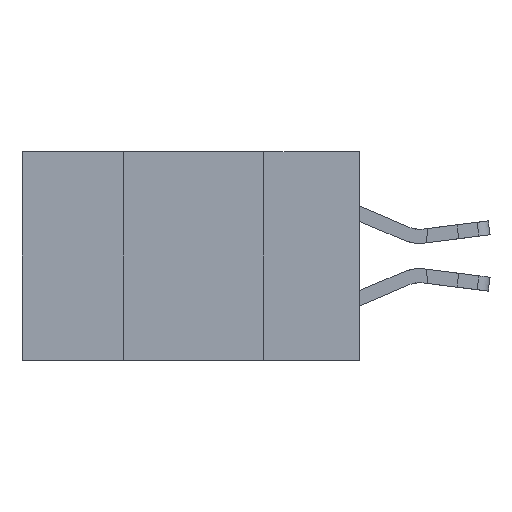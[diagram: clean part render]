
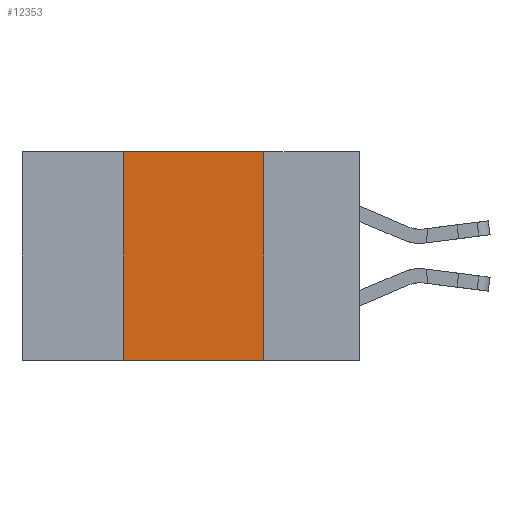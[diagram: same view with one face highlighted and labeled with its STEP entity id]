
A CAD part, left-side view. The second image highlights one B-rep face of the part: STEP entity #12353.
In plain terms, the highlighted planar face has unit normal (-1, 0, 0).
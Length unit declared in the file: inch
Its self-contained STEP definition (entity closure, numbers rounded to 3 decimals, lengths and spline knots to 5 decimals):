
#75 = ORIENTED_EDGE ( 'NONE', *, *, #1564, .F. ) ;
#1560 = AXIS2_PLACEMENT_3D ( 'NONE', #17747, #12149, #10774 ) ;
#1564 = EDGE_CURVE ( 'NONE', #12366, #2827, #11663, .T. ) ;
#2827 = VERTEX_POINT ( 'NONE', #4999 ) ;
#3298 = CARTESIAN_POINT ( 'NONE',  ( 0., 0.6, -0.37 ) ) ;
#3664 = CARTESIAN_POINT ( 'NONE',  ( 0., 0.42, 0. ) ) ;
#4999 = CARTESIAN_POINT ( 'NONE',  ( 0., 0.42, 0. ) ) ;
#5420 = CARTESIAN_POINT ( 'NONE',  ( 0., 0.17, 0. ) ) ;
#5741 = VECTOR ( 'NONE', #18306, 39.37008 ) ;
#5853 = EDGE_LOOP ( 'NONE', ( #17055, #16620, #75, #18424 ) ) ;
#5972 = EDGE_CURVE ( 'NONE', #16258, #6497, #9578, .T. ) ;
#6440 = PLANE ( 'NONE',  #1560 ) ;
#6497 = VERTEX_POINT ( 'NONE', #16354 ) ;
#8377 = LINE ( 'NONE', #3298, #9045 ) ;
#8579 = EDGE_CURVE ( 'NONE', #12366, #6497, #8377, .T. ) ;
#9045 = VECTOR ( 'NONE', #11683, 39.37008 ) ;
#9398 = CARTESIAN_POINT ( 'NONE',  ( 0., 0.42, -0.37 ) ) ;
#9578 = LINE ( 'NONE', #5420, #5741 ) ;
#9672 = VECTOR ( 'NONE', #12308, 39.37008 ) ;
#10774 = DIRECTION ( 'NONE',  ( 0., 0., -1. ) ) ;
#11289 = VECTOR ( 'NONE', #15701, 39.37008 ) ;
#11663 = LINE ( 'NONE', #3664, #9672 ) ;
#11683 = DIRECTION ( 'NONE',  ( 0., -1., 0. ) ) ;
#12149 = DIRECTION ( 'NONE',  ( 1., 0., 0. ) ) ;
#12308 = DIRECTION ( 'NONE',  ( 0., 0., 1. ) ) ;
#12353 = ADVANCED_FACE ( 'NONE', ( #14405 ), #6440, .F. ) ;
#12366 = VERTEX_POINT ( 'NONE', #9398 ) ;
#12898 = EDGE_CURVE ( 'NONE', #2827, #16258, #16832, .T. ) ;
#14405 = FACE_OUTER_BOUND ( 'NONE', #5853, .T. ) ;
#14499 = CARTESIAN_POINT ( 'NONE',  ( 0., 0.6, 0. ) ) ;
#15701 = DIRECTION ( 'NONE',  ( 0., -1., 0. ) ) ;
#16258 = VERTEX_POINT ( 'NONE', #17393 ) ;
#16354 = CARTESIAN_POINT ( 'NONE',  ( 0., 0.17, -0.37 ) ) ;
#16620 = ORIENTED_EDGE ( 'NONE', *, *, #12898, .F. ) ;
#16832 = LINE ( 'NONE', #14499, #11289 ) ;
#17055 = ORIENTED_EDGE ( 'NONE', *, *, #5972, .F. ) ;
#17393 = CARTESIAN_POINT ( 'NONE',  ( 0., 0.17, 0. ) ) ;
#17747 = CARTESIAN_POINT ( 'NONE',  ( 0., 0.6, 0. ) ) ;
#18306 = DIRECTION ( 'NONE',  ( 0., 0., -1. ) ) ;
#18424 = ORIENTED_EDGE ( 'NONE', *, *, #8579, .T. ) ;
